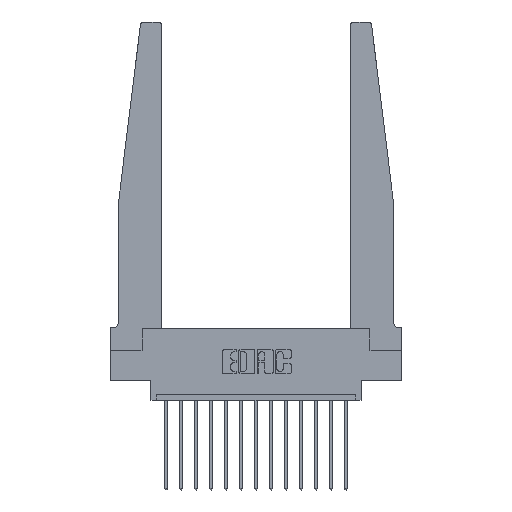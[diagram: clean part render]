
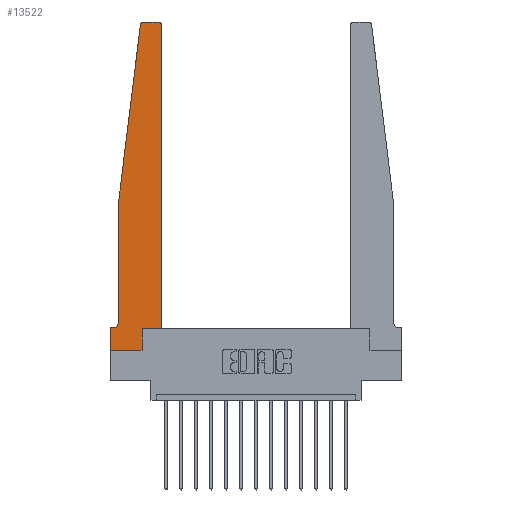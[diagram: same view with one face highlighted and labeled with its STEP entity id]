
A CAD part, top view. The second image highlights one B-rep face of the part: STEP entity #13522.
In plain terms, the highlighted planar face has unit normal (0, 0, 1).
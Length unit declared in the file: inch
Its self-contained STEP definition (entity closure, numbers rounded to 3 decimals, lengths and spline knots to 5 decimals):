
#108 = CARTESIAN_POINT ( 'NONE',  ( 0., 0., 0.37 ) ) ;
#115 = VECTOR ( 'NONE', #3883, 39.37008 ) ;
#252 = AXIS2_PLACEMENT_3D ( 'NONE', #15372, #16693, #9954 ) ;
#289 = EDGE_CURVE ( 'NONE', #5541, #8992, #15062, .T. ) ;
#365 = CIRCLE ( 'NONE', #12954, 0.03 ) ;
#470 = LINE ( 'NONE', #15338, #1501 ) ;
#636 = CARTESIAN_POINT ( 'NONE',  ( 0.065, 0.1875, 0.37 ) ) ;
#712 = VERTEX_POINT ( 'NONE', #15443 ) ;
#775 = LINE ( 'NONE', #12595, #4841 ) ;
#985 = ORIENTED_EDGE ( 'NONE', *, *, #4553, .T. ) ;
#1000 = EDGE_CURVE ( 'NONE', #8017, #2411, #15251, .T. ) ;
#1056 = EDGE_CURVE ( 'NONE', #8992, #12667, #16477, .T. ) ;
#1218 = DIRECTION ( 'NONE',  ( 0., 0., 1. ) ) ;
#1250 = LINE ( 'NONE', #5205, #115 ) ;
#1426 = CARTESIAN_POINT ( 'NONE',  ( 0.065, 1.25, 0.37 ) ) ;
#1501 = VECTOR ( 'NONE', #11322, 39.37008 ) ;
#1644 = LINE ( 'NONE', #4373, #6787 ) ;
#1824 = DIRECTION ( 'NONE',  ( 0., 1., 0. ) ) ;
#1861 = DIRECTION ( 'NONE',  ( -1., 0., 0. ) ) ;
#2074 = ORIENTED_EDGE ( 'NONE', *, *, #9399, .T. ) ;
#2411 = VERTEX_POINT ( 'NONE', #7539 ) ;
#2998 = DIRECTION ( 'NONE',  ( 0., 0., 1. ) ) ;
#3145 = CIRCLE ( 'NONE', #13226, 0.03 ) ;
#3265 = CARTESIAN_POINT ( 'NONE',  ( 0., 0., 0.37 ) ) ;
#3555 = VERTEX_POINT ( 'NONE', #17267 ) ;
#3827 = DIRECTION ( 'NONE',  ( 0., 0., 1. ) ) ;
#3883 = DIRECTION ( 'NONE',  ( -1., 0., 0. ) ) ;
#4075 = LINE ( 'NONE', #1426, #4132 ) ;
#4132 = VECTOR ( 'NONE', #9134, 39.37008 ) ;
#4186 = ORIENTED_EDGE ( 'NONE', *, *, #14102, .T. ) ;
#4290 = ORIENTED_EDGE ( 'NONE', *, *, #5486, .T. ) ;
#4373 = CARTESIAN_POINT ( 'NONE',  ( 0.2605, 0.18, 0.37 ) ) ;
#4553 = EDGE_CURVE ( 'NONE', #712, #15296, #365, .T. ) ;
#4841 = VECTOR ( 'NONE', #16883, 39.37008 ) ;
#4856 = ORIENTED_EDGE ( 'NONE', *, *, #289, .T. ) ;
#4867 = LINE ( 'NONE', #6174, #10953 ) ;
#4980 = ORIENTED_EDGE ( 'NONE', *, *, #17278, .T. ) ;
#5205 = CARTESIAN_POINT ( 'NONE',  ( 0.25, 2.75, 0.37 ) ) ;
#5299 = CARTESIAN_POINT ( 'NONE',  ( 0.24675, 2.72367, 0.37 ) ) ;
#5486 = EDGE_CURVE ( 'NONE', #5561, #3555, #4075, .T. ) ;
#5541 = VERTEX_POINT ( 'NONE', #7824 ) ;
#5561 = VERTEX_POINT ( 'NONE', #5299 ) ;
#5976 = VERTEX_POINT ( 'NONE', #16285 ) ;
#6174 = CARTESIAN_POINT ( 'NONE',  ( 0.425, 0.18, 0.37 ) ) ;
#6367 = CARTESIAN_POINT ( 'NONE',  ( 0.27653, 2.72, 0.37 ) ) ;
#6652 = CARTESIAN_POINT ( 'NONE',  ( 0., 0.1875, 0.37 ) ) ;
#6787 = VECTOR ( 'NONE', #1824, 39.37008 ) ;
#6981 = VECTOR ( 'NONE', #13854, 39.37008 ) ;
#7132 = EDGE_LOOP ( 'NONE', ( #4980, #2074, #4290, #13114, #4856, #15732, #13768, #15912, #16422, #4186, #11329, #985 ) ) ;
#7539 = CARTESIAN_POINT ( 'NONE',  ( 0.2605, 0., 0.37 ) ) ;
#7557 = DIRECTION ( 'NONE',  ( 1., 0., 0. ) ) ;
#7579 = CARTESIAN_POINT ( 'NONE',  ( 0.065, 1.25, 0.37 ) ) ;
#7824 = CARTESIAN_POINT ( 'NONE',  ( 0.065, 0.2375, 0.37 ) ) ;
#8017 = VERTEX_POINT ( 'NONE', #108 ) ;
#8127 = PLANE ( 'NONE',  #13455 ) ;
#8992 = VERTEX_POINT ( 'NONE', #13384 ) ;
#9134 = DIRECTION ( 'NONE',  ( -0.122, -0.992, 0. ) ) ;
#9244 = CARTESIAN_POINT ( 'NONE',  ( 0.425, 0.18, 0.37 ) ) ;
#9352 = DIRECTION ( 'NONE',  ( 1., 0., 0. ) ) ;
#9399 = EDGE_CURVE ( 'NONE', #17256, #5561, #3145, .T. ) ;
#9954 = DIRECTION ( 'NONE',  ( -1., 0., 0. ) ) ;
#10346 = EDGE_CURVE ( 'NONE', #2411, #5976, #1644, .T. ) ;
#10534 = VERTEX_POINT ( 'NONE', #9244 ) ;
#10937 = EDGE_CURVE ( 'NONE', #10534, #712, #775, .T. ) ;
#10953 = VECTOR ( 'NONE', #7557, 39.37008 ) ;
#11322 = DIRECTION ( 'NONE',  ( 0., -1., 0. ) ) ;
#11329 = ORIENTED_EDGE ( 'NONE', *, *, #10937, .T. ) ;
#11615 = LINE ( 'NONE', #7579, #12615 ) ;
#12595 = CARTESIAN_POINT ( 'NONE',  ( 0.425, 0.18, 0.37 ) ) ;
#12615 = VECTOR ( 'NONE', #14227, 39.37008 ) ;
#12667 = VERTEX_POINT ( 'NONE', #12756 ) ;
#12756 = CARTESIAN_POINT ( 'NONE',  ( 0., 0.1875, 0.37 ) ) ;
#12954 = AXIS2_PLACEMENT_3D ( 'NONE', #14990, #2998, #14025 ) ;
#13111 = VECTOR ( 'NONE', #1861, 39.37008 ) ;
#13114 = ORIENTED_EDGE ( 'NONE', *, *, #13734, .T. ) ;
#13226 = AXIS2_PLACEMENT_3D ( 'NONE', #6367, #3827, #17031 ) ;
#13384 = CARTESIAN_POINT ( 'NONE',  ( 0.015, 0.1875, 0.37 ) ) ;
#13455 = AXIS2_PLACEMENT_3D ( 'NONE', #6652, #1218, #9352 ) ;
#13522 = ADVANCED_FACE ( 'NONE', ( #17247 ), #8127, .T. ) ;
#13734 = EDGE_CURVE ( 'NONE', #3555, #5541, #11615, .T. ) ;
#13768 = ORIENTED_EDGE ( 'NONE', *, *, #17132, .T. ) ;
#13854 = DIRECTION ( 'NONE',  ( 1., 0., 0. ) ) ;
#14025 = DIRECTION ( 'NONE',  ( 1., 0., 0. ) ) ;
#14102 = EDGE_CURVE ( 'NONE', #5976, #10534, #4867, .T. ) ;
#14227 = DIRECTION ( 'NONE',  ( 0., -1., 0. ) ) ;
#14452 = CARTESIAN_POINT ( 'NONE',  ( 0.27653, 2.75, 0.37 ) ) ;
#14990 = CARTESIAN_POINT ( 'NONE',  ( 0.395, 2.72, 0.37 ) ) ;
#15062 = CIRCLE ( 'NONE', #252, 0.05 ) ;
#15251 = LINE ( 'NONE', #3265, #6981 ) ;
#15296 = VERTEX_POINT ( 'NONE', #15726 ) ;
#15338 = CARTESIAN_POINT ( 'NONE',  ( 0., 0., 0.37 ) ) ;
#15372 = CARTESIAN_POINT ( 'NONE',  ( 0.015, 0.2375, 0.37 ) ) ;
#15443 = CARTESIAN_POINT ( 'NONE',  ( 0.425, 2.72, 0.37 ) ) ;
#15726 = CARTESIAN_POINT ( 'NONE',  ( 0.395, 2.75, 0.37 ) ) ;
#15732 = ORIENTED_EDGE ( 'NONE', *, *, #1056, .T. ) ;
#15912 = ORIENTED_EDGE ( 'NONE', *, *, #1000, .T. ) ;
#16285 = CARTESIAN_POINT ( 'NONE',  ( 0.2605, 0.18, 0.37 ) ) ;
#16422 = ORIENTED_EDGE ( 'NONE', *, *, #10346, .T. ) ;
#16477 = LINE ( 'NONE', #636, #13111 ) ;
#16693 = DIRECTION ( 'NONE',  ( 0., 0., -1. ) ) ;
#16883 = DIRECTION ( 'NONE',  ( 0., 1., 0. ) ) ;
#17031 = DIRECTION ( 'NONE',  ( 1., 0., 0. ) ) ;
#17132 = EDGE_CURVE ( 'NONE', #12667, #8017, #470, .T. ) ;
#17247 = FACE_OUTER_BOUND ( 'NONE', #7132, .T. ) ;
#17256 = VERTEX_POINT ( 'NONE', #14452 ) ;
#17267 = CARTESIAN_POINT ( 'NONE',  ( 0.065, 1.25, 0.37 ) ) ;
#17278 = EDGE_CURVE ( 'NONE', #15296, #17256, #1250, .T. ) ;
